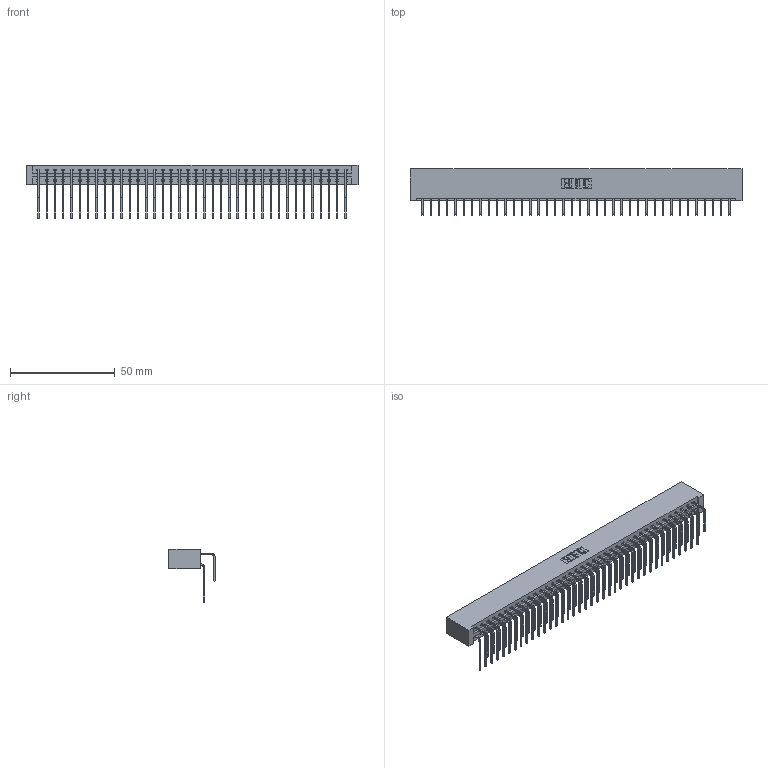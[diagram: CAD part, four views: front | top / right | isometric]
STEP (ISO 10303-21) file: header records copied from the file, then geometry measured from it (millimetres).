
FILE_DESCRIPTION (( 'STEP AP203' ), '1' );
FILE_NAME ('387-076-558-201.STEP', '2018-09-23T16:12:02', ( '' ), ( '' ), 'SwSTEP 2.0', 'SolidWorks 2016', '' );
FILE_SCHEMA (( 'CONFIG_CONTROL_DESIGN' ));
Length unit declared in the file: inch
Products named in the file (4): 387-076-558-201; 337 Part_No Mounting Lugs; 345-292-001_558 559 Tail - 1; 345-292-001_558 Tail - 2
Assembly tree (77 placements, depth 2):
  387-076-558-201
    337 Part_No Mounting Lugs
    345-292-001_558 559 Tail - 1  x38
    345-292-001_558 Tail - 2  x38
Bounding box: 158.45 x 22.17 x 25.53 mm (x, y, z)
Volume: 17844.1 mm3; surface area: 22391.5 mm2
Topology: 77 solids, 77 shells, 4362 faces, 12979 edges, 8550 vertices
Faces by surface type: plane 3106, cylinder 1256
Entity records: 31487 total; most frequent: CARTESIAN_POINT 5353, ORIENTED_EDGE 5238, DIRECTION 4535, EDGE_CURVE 2619, VECTOR 2459, LINE 2459, VERTEX_POINT 1742, AXIS2_PLACEMENT_3D 1038
